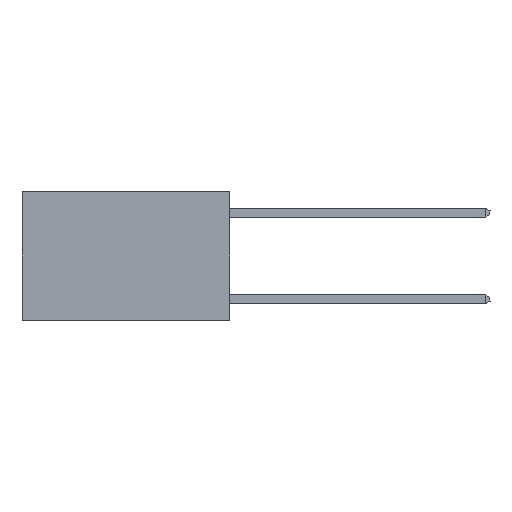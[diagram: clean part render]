
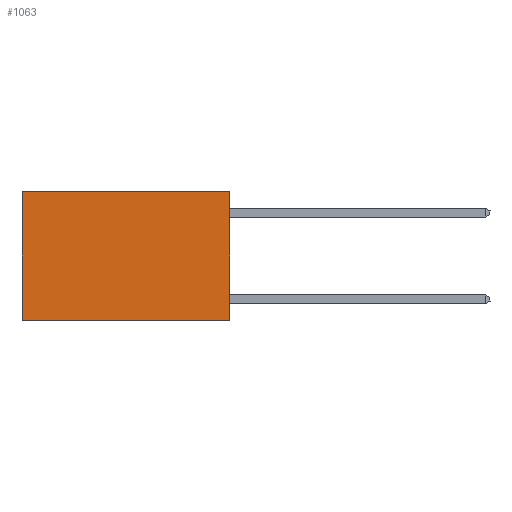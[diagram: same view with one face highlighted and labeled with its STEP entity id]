
A CAD part, left-side view. The second image highlights one B-rep face of the part: STEP entity #1063.
In plain terms, the highlighted planar face has unit normal (-1, 0, 0).
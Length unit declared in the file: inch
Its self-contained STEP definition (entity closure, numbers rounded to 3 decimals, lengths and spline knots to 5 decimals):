
#137 = EDGE_CURVE ( 'NONE', #3541, #5506, #404, .T. ) ;
#402 = VECTOR ( 'NONE', #6741, 39.37008 ) ;
#404 = LINE ( 'NONE', #4699, #3413 ) ;
#776 = EDGE_LOOP ( 'NONE', ( #5875, #7794, #7527, #3056 ) ) ;
#810 = CARTESIAN_POINT ( 'NONE',  ( 0.2625, 0., -0.37 ) ) ;
#984 = LINE ( 'NONE', #8013, #402 ) ;
#1063 = ADVANCED_FACE ( 'NONE', ( #1733 ), #6065, .F. ) ;
#1733 = FACE_OUTER_BOUND ( 'NONE', #776, .T. ) ;
#2032 = LINE ( 'NONE', #7563, #6263 ) ;
#2468 = DIRECTION ( 'NONE',  ( 0., 0., -1. ) ) ;
#2672 = CARTESIAN_POINT ( 'NONE',  ( 0.2625, 0.6, 0. ) ) ;
#2770 = DIRECTION ( 'NONE',  ( 0., 0., -1. ) ) ;
#2820 = LINE ( 'NONE', #3544, #8974 ) ;
#3056 = ORIENTED_EDGE ( 'NONE', *, *, #3335, .T. ) ;
#3192 = EDGE_CURVE ( 'NONE', #5856, #5506, #2820, .T. ) ;
#3335 = EDGE_CURVE ( 'NONE', #7621, #3541, #984, .T. ) ;
#3413 = VECTOR ( 'NONE', #6098, 39.37008 ) ;
#3541 = VERTEX_POINT ( 'NONE', #2672 ) ;
#3544 = CARTESIAN_POINT ( 'NONE',  ( 0.2625, 0., -0.37 ) ) ;
#4512 = CARTESIAN_POINT ( 'NONE',  ( 0.2625, 0.6, -0.37 ) ) ;
#4699 = CARTESIAN_POINT ( 'NONE',  ( 0.2625, 0.6, 0. ) ) ;
#5325 = DIRECTION ( 'NONE',  ( 1., 0., 0. ) ) ;
#5506 = VERTEX_POINT ( 'NONE', #4512 ) ;
#5731 = EDGE_CURVE ( 'NONE', #7621, #5856, #2032, .T. ) ;
#5856 = VERTEX_POINT ( 'NONE', #810 ) ;
#5875 = ORIENTED_EDGE ( 'NONE', *, *, #137, .T. ) ;
#6065 = PLANE ( 'NONE',  #6593 ) ;
#6098 = DIRECTION ( 'NONE',  ( 0., 0., -1. ) ) ;
#6263 = VECTOR ( 'NONE', #2770, 39.37008 ) ;
#6573 = CARTESIAN_POINT ( 'NONE',  ( 0.2625, 0., 0. ) ) ;
#6593 = AXIS2_PLACEMENT_3D ( 'NONE', #6573, #5325, #2468 ) ;
#6741 = DIRECTION ( 'NONE',  ( 0., 1., 0. ) ) ;
#7197 = DIRECTION ( 'NONE',  ( 0., 1., 0. ) ) ;
#7346 = CARTESIAN_POINT ( 'NONE',  ( 0.2625, 0., 0. ) ) ;
#7527 = ORIENTED_EDGE ( 'NONE', *, *, #5731, .F. ) ;
#7563 = CARTESIAN_POINT ( 'NONE',  ( 0.2625, 0., 0. ) ) ;
#7621 = VERTEX_POINT ( 'NONE', #7346 ) ;
#7794 = ORIENTED_EDGE ( 'NONE', *, *, #3192, .F. ) ;
#8013 = CARTESIAN_POINT ( 'NONE',  ( 0.2625, 0., 0. ) ) ;
#8974 = VECTOR ( 'NONE', #7197, 39.37008 ) ;
